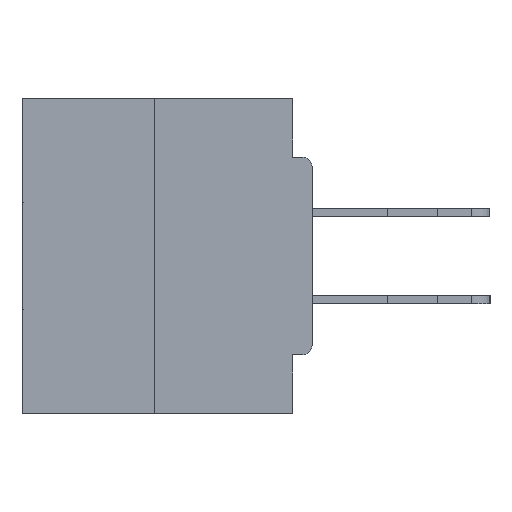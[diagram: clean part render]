
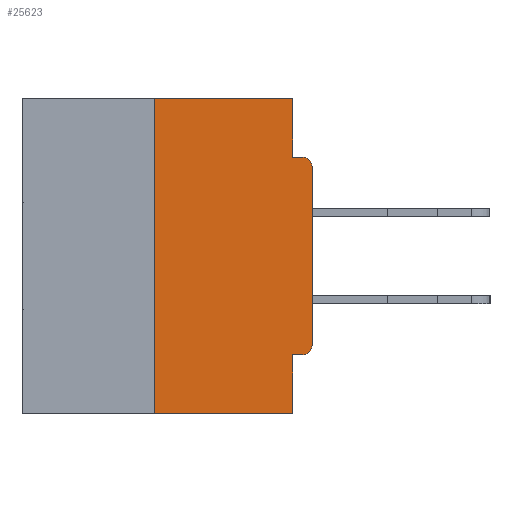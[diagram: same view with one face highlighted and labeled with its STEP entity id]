
A CAD part, left-side view. The second image highlights one B-rep face of the part: STEP entity #25623.
In plain terms, the highlighted planar face has unit normal (-1, 0, 0).
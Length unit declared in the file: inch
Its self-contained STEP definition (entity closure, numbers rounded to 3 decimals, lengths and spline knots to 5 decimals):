
#939 = FACE_OUTER_BOUND ( 'NONE', #19822, .T. ) ;
#1061 = LINE ( 'NONE', #29066, #15677 ) ;
#1254 = DIRECTION ( 'NONE',  ( -1., 0., 0. ) ) ;
#2058 = AXIS2_PLACEMENT_3D ( 'NONE', #23729, #30089, #9683 ) ;
#2145 = ORIENTED_EDGE ( 'NONE', *, *, #16097, .F. ) ;
#2354 = VECTOR ( 'NONE', #17868, 39.37008 ) ;
#2956 = LINE ( 'NONE', #15483, #9799 ) ;
#3666 = CARTESIAN_POINT ( 'NONE',  ( 0., 0.031, -0.0935 ) ) ;
#3677 = CARTESIAN_POINT ( 'NONE',  ( 0., 0., -0.3915 ) ) ;
#3755 = DIRECTION ( 'NONE',  ( 0., 1., 0. ) ) ;
#4337 = DIRECTION ( 'NONE',  ( 0., 0., -1. ) ) ;
#5664 = VERTEX_POINT ( 'NONE', #36866 ) ;
#5862 = EDGE_CURVE ( 'NONE', #28731, #5664, #7352, .T. ) ;
#6015 = EDGE_CURVE ( 'NONE', #28731, #21323, #14564, .T. ) ;
#6415 = CARTESIAN_POINT ( 'NONE',  ( 0., 0.015, -0.4065 ) ) ;
#6807 = AXIS2_PLACEMENT_3D ( 'NONE', #18868, #33653, #4337 ) ;
#6872 = VECTOR ( 'NONE', #8247, 39.37008 ) ;
#7001 = DIRECTION ( 'NONE',  ( 0., 0., -1. ) ) ;
#7128 = CARTESIAN_POINT ( 'NONE',  ( 0., 0.46, 0. ) ) ;
#7352 = LINE ( 'NONE', #29303, #19630 ) ;
#8247 = DIRECTION ( 'NONE',  ( 0., -1., 0. ) ) ;
#8406 = ORIENTED_EDGE ( 'NONE', *, *, #11970, .F. ) ;
#9683 = DIRECTION ( 'NONE',  ( 0., 0., -1. ) ) ;
#9799 = VECTOR ( 'NONE', #3755, 39.37008 ) ;
#11163 = CARTESIAN_POINT ( 'NONE',  ( 0., 0.46, -0.5 ) ) ;
#11469 = ORIENTED_EDGE ( 'NONE', *, *, #33738, .T. ) ;
#11970 = EDGE_CURVE ( 'NONE', #5664, #18525, #30229, .T. ) ;
#12606 = LINE ( 'NONE', #29550, #28111 ) ;
#12750 = EDGE_CURVE ( 'NONE', #18525, #29119, #27447, .T. ) ;
#12945 = VERTEX_POINT ( 'NONE', #29457 ) ;
#13218 = ORIENTED_EDGE ( 'NONE', *, *, #16638, .F. ) ;
#14347 = ORIENTED_EDGE ( 'NONE', *, *, #17365, .F. ) ;
#14564 = LINE ( 'NONE', #11163, #6872 ) ;
#14877 = DIRECTION ( 'NONE',  ( 0., 0., 1. ) ) ;
#15112 = ORIENTED_EDGE ( 'NONE', *, *, #5862, .F. ) ;
#15483 = CARTESIAN_POINT ( 'NONE',  ( 0., 0., -0.4065 ) ) ;
#15677 = VECTOR ( 'NONE', #29312, 39.37008 ) ;
#15701 = EDGE_CURVE ( 'NONE', #18401, #16067, #29974, .T. ) ;
#15973 = VERTEX_POINT ( 'NONE', #31570 ) ;
#16067 = VERTEX_POINT ( 'NONE', #3677 ) ;
#16097 = EDGE_CURVE ( 'NONE', #29119, #25266, #12606, .T. ) ;
#16638 = EDGE_CURVE ( 'NONE', #18401, #12945, #2956, .T. ) ;
#16732 = VECTOR ( 'NONE', #14877, 39.37008 ) ;
#17365 = EDGE_CURVE ( 'NONE', #12945, #21323, #1061, .T. ) ;
#17868 = DIRECTION ( 'NONE',  ( 0., 0., -1. ) ) ;
#18401 = VERTEX_POINT ( 'NONE', #6415 ) ;
#18525 = VERTEX_POINT ( 'NONE', #30001 ) ;
#18547 = ORIENTED_EDGE ( 'NONE', *, *, #12750, .F. ) ;
#18868 = CARTESIAN_POINT ( 'NONE',  ( 0., 0.46, 0. ) ) ;
#19036 = CARTESIAN_POINT ( 'NONE',  ( 0., 0.015, -0.0935 ) ) ;
#19630 = VECTOR ( 'NONE', #32244, 39.37008 ) ;
#19822 = EDGE_LOOP ( 'NONE', ( #8406, #15112, #23060, #14347, #13218, #24903, #11469, #36873, #2145, #18547 ) ) ;
#20904 = DIRECTION ( 'NONE',  ( 0., -1., 0. ) ) ;
#21323 = VERTEX_POINT ( 'NONE', #34158 ) ;
#23060 = ORIENTED_EDGE ( 'NONE', *, *, #6015, .T. ) ;
#23729 = CARTESIAN_POINT ( 'NONE',  ( 0., 0.015, -0.3915 ) ) ;
#24507 = LINE ( 'NONE', #26498, #16732 ) ;
#24903 = ORIENTED_EDGE ( 'NONE', *, *, #15701, .T. ) ;
#25266 = VERTEX_POINT ( 'NONE', #19036 ) ;
#25623 = ADVANCED_FACE ( 'NONE', ( #939 ), #36313, .F. ) ;
#26115 = VECTOR ( 'NONE', #33370, 39.37008 ) ;
#26498 = CARTESIAN_POINT ( 'NONE',  ( 0., 0., 0. ) ) ;
#26597 = AXIS2_PLACEMENT_3D ( 'NONE', #35912, #1254, #7001 ) ;
#27447 = LINE ( 'NONE', #32005, #2354 ) ;
#28111 = VECTOR ( 'NONE', #20904, 39.37008 ) ;
#28731 = VERTEX_POINT ( 'NONE', #29638 ) ;
#29066 = CARTESIAN_POINT ( 'NONE',  ( 0., 0.031, -0.5 ) ) ;
#29119 = VERTEX_POINT ( 'NONE', #3666 ) ;
#29303 = CARTESIAN_POINT ( 'NONE',  ( 0., 0.25, 0. ) ) ;
#29312 = DIRECTION ( 'NONE',  ( 0., 0., -1. ) ) ;
#29457 = CARTESIAN_POINT ( 'NONE',  ( 0., 0.031, -0.4065 ) ) ;
#29550 = CARTESIAN_POINT ( 'NONE',  ( 0., 0., -0.0935 ) ) ;
#29638 = CARTESIAN_POINT ( 'NONE',  ( 0., 0.25, -0.5 ) ) ;
#29974 = CIRCLE ( 'NONE', #2058, 0.015 ) ;
#30001 = CARTESIAN_POINT ( 'NONE',  ( 0., 0.031, 0. ) ) ;
#30089 = DIRECTION ( 'NONE',  ( -1., 0., 0. ) ) ;
#30229 = LINE ( 'NONE', #7128, #26115 ) ;
#31570 = CARTESIAN_POINT ( 'NONE',  ( 0., 0., -0.1085 ) ) ;
#32005 = CARTESIAN_POINT ( 'NONE',  ( 0., 0.031, 0. ) ) ;
#32244 = DIRECTION ( 'NONE',  ( 0., 0., 1. ) ) ;
#32466 = CIRCLE ( 'NONE', #26597, 0.015 ) ;
#33370 = DIRECTION ( 'NONE',  ( 0., -1., 0. ) ) ;
#33653 = DIRECTION ( 'NONE',  ( 1., 0., 0. ) ) ;
#33738 = EDGE_CURVE ( 'NONE', #16067, #15973, #24507, .T. ) ;
#34158 = CARTESIAN_POINT ( 'NONE',  ( 0., 0.031, -0.5 ) ) ;
#35912 = CARTESIAN_POINT ( 'NONE',  ( 0., 0.015, -0.1085 ) ) ;
#36313 = PLANE ( 'NONE',  #6807 ) ;
#36527 = EDGE_CURVE ( 'NONE', #15973, #25266, #32466, .T. ) ;
#36866 = CARTESIAN_POINT ( 'NONE',  ( 0., 0.25, 0. ) ) ;
#36873 = ORIENTED_EDGE ( 'NONE', *, *, #36527, .T. ) ;
